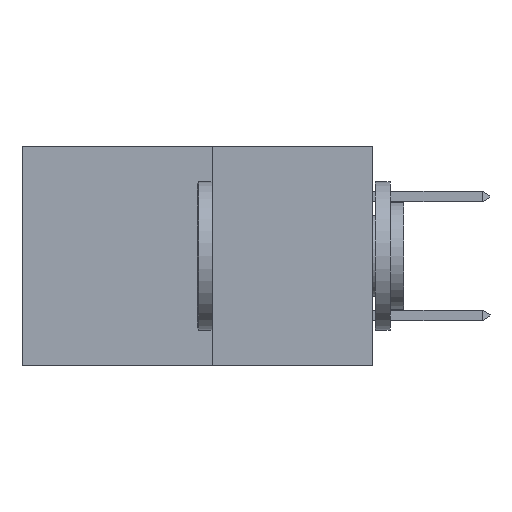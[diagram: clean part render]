
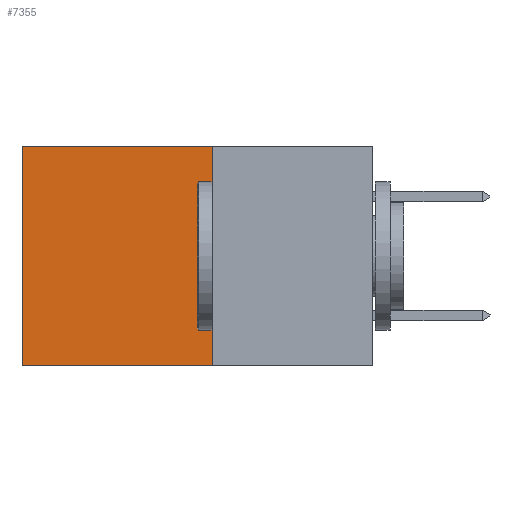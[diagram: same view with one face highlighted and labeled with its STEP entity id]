
A CAD part, left-side view. The second image highlights one B-rep face of the part: STEP entity #7355.
In plain terms, the highlighted planar face has unit normal (-1, 0, 0).
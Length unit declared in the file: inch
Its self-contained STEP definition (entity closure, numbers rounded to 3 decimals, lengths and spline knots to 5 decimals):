
#5 = LINE ( 'NONE', #3280, #5378 ) ;
#655 = CARTESIAN_POINT ( 'NONE',  ( 0.277, 0.27, 0. ) ) ;
#1096 = DIRECTION ( 'NONE',  ( 0., 1., 0. ) ) ;
#1098 = VECTOR ( 'NONE', #2691, 39.37008 ) ;
#1488 = LINE ( 'NONE', #2559, #3096 ) ;
#1711 = ORIENTED_EDGE ( 'NONE', *, *, #3870, .T. ) ;
#1917 = FACE_OUTER_BOUND ( 'NONE', #4485, .T. ) ;
#1969 = CARTESIAN_POINT ( 'NONE',  ( 0.277, 0.59, -0.37 ) ) ;
#2286 = ORIENTED_EDGE ( 'NONE', *, *, #6080, .F. ) ;
#2501 = LINE ( 'NONE', #5690, #4200 ) ;
#2559 = CARTESIAN_POINT ( 'NONE',  ( 0.277, 0.27, -0.37 ) ) ;
#2589 = VERTEX_POINT ( 'NONE', #8294 ) ;
#2670 = PLANE ( 'NONE',  #6707 ) ;
#2691 = DIRECTION ( 'NONE',  ( 0., 0., -1. ) ) ;
#2879 = ORIENTED_EDGE ( 'NONE', *, *, #5581, .F. ) ;
#3096 = VECTOR ( 'NONE', #7993, 39.37008 ) ;
#3280 = CARTESIAN_POINT ( 'NONE',  ( 0.277, 0.27, -0.37 ) ) ;
#3368 = ORIENTED_EDGE ( 'NONE', *, *, #3506, .T. ) ;
#3381 = DIRECTION ( 'NONE',  ( 1., 0., 0. ) ) ;
#3506 = EDGE_CURVE ( 'NONE', #8598, #3922, #2501, .T. ) ;
#3870 = EDGE_CURVE ( 'NONE', #3922, #8272, #8283, .T. ) ;
#3922 = VERTEX_POINT ( 'NONE', #6205 ) ;
#4022 = DIRECTION ( 'NONE',  ( 0., 1., 0. ) ) ;
#4200 = VECTOR ( 'NONE', #1096, 39.37008 ) ;
#4485 = EDGE_LOOP ( 'NONE', ( #1711, #2879, #2286, #3368 ) ) ;
#5378 = VECTOR ( 'NONE', #4022, 39.37008 ) ;
#5432 = CARTESIAN_POINT ( 'NONE',  ( 0.277, 0.59, -0.37 ) ) ;
#5581 = EDGE_CURVE ( 'NONE', #2589, #8272, #5, .T. ) ;
#5690 = CARTESIAN_POINT ( 'NONE',  ( 0.277, 0.27, 0. ) ) ;
#6080 = EDGE_CURVE ( 'NONE', #8598, #2589, #1488, .T. ) ;
#6200 = CARTESIAN_POINT ( 'NONE',  ( 0.277, 0.27, -0.37 ) ) ;
#6205 = CARTESIAN_POINT ( 'NONE',  ( 0.277, 0.59, 0. ) ) ;
#6707 = AXIS2_PLACEMENT_3D ( 'NONE', #6200, #3381, #8081 ) ;
#7355 = ADVANCED_FACE ( 'NONE', ( #1917 ), #2670, .F. ) ;
#7993 = DIRECTION ( 'NONE',  ( 0., 0., -1. ) ) ;
#8081 = DIRECTION ( 'NONE',  ( 0., 0., -1. ) ) ;
#8272 = VERTEX_POINT ( 'NONE', #1969 ) ;
#8283 = LINE ( 'NONE', #5432, #1098 ) ;
#8294 = CARTESIAN_POINT ( 'NONE',  ( 0.277, 0.27, -0.37 ) ) ;
#8598 = VERTEX_POINT ( 'NONE', #655 ) ;
